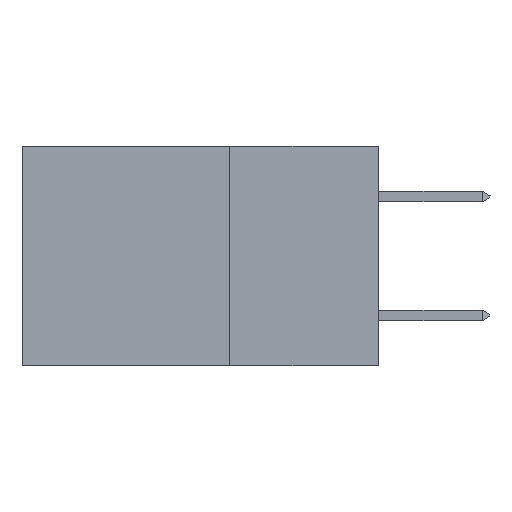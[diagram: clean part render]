
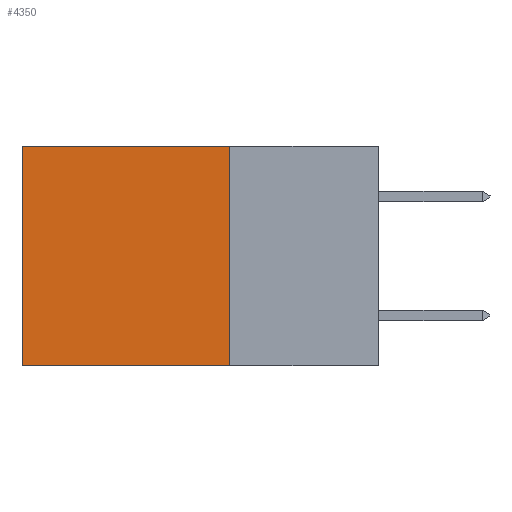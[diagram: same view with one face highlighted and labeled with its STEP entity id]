
A CAD part, left-side view. The second image highlights one B-rep face of the part: STEP entity #4350.
In plain terms, the highlighted planar face has unit normal (-1, 0, 0).
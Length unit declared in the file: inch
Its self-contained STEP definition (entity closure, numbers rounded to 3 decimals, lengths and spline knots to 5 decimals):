
#243 = EDGE_CURVE ( 'NONE', #7638, #7333, #8550, .T. ) ;
#1134 = LINE ( 'NONE', #7123, #10277 ) ;
#1399 = VERTEX_POINT ( 'NONE', #10328 ) ;
#1833 = EDGE_LOOP ( 'NONE', ( #2424, #3683, #6592, #6654 ) ) ;
#2219 = CARTESIAN_POINT ( 'NONE',  ( 0.2615, 0.25, -0.37 ) ) ;
#2424 = ORIENTED_EDGE ( 'NONE', *, *, #12618, .T. ) ;
#2612 = DIRECTION ( 'NONE',  ( 0., 1., 0. ) ) ;
#3199 = AXIS2_PLACEMENT_3D ( 'NONE', #2219, #3296, #6269 ) ;
#3251 = EDGE_CURVE ( 'NONE', #11670, #1399, #8200, .T. ) ;
#3296 = DIRECTION ( 'NONE',  ( 1., 0., 0. ) ) ;
#3599 = CARTESIAN_POINT ( 'NONE',  ( 0.2615, 0.25, -0.37 ) ) ;
#3664 = LINE ( 'NONE', #12708, #12023 ) ;
#3683 = ORIENTED_EDGE ( 'NONE', *, *, #243, .F. ) ;
#4350 = ADVANCED_FACE ( 'NONE', ( #5340 ), #7191, .F. ) ;
#5340 = FACE_OUTER_BOUND ( 'NONE', #1833, .T. ) ;
#6269 = DIRECTION ( 'NONE',  ( 0., 0., -1. ) ) ;
#6452 = EDGE_CURVE ( 'NONE', #11670, #7638, #3664, .T. ) ;
#6592 = ORIENTED_EDGE ( 'NONE', *, *, #6452, .F. ) ;
#6654 = ORIENTED_EDGE ( 'NONE', *, *, #3251, .T. ) ;
#7123 = CARTESIAN_POINT ( 'NONE',  ( 0.2615, 0.6, -0.37 ) ) ;
#7191 = PLANE ( 'NONE',  #3199 ) ;
#7274 = DIRECTION ( 'NONE',  ( 0., 1., 0. ) ) ;
#7333 = VERTEX_POINT ( 'NONE', #12725 ) ;
#7638 = VERTEX_POINT ( 'NONE', #12649 ) ;
#8139 = CARTESIAN_POINT ( 'NONE',  ( 0.2615, 0.25, 0. ) ) ;
#8200 = LINE ( 'NONE', #8139, #9602 ) ;
#8271 = CARTESIAN_POINT ( 'NONE',  ( 0.2615, 0.25, 0. ) ) ;
#8546 = DIRECTION ( 'NONE',  ( 0., 0., -1. ) ) ;
#8550 = LINE ( 'NONE', #3599, #11061 ) ;
#9349 = DIRECTION ( 'NONE',  ( 0., 0., -1. ) ) ;
#9602 = VECTOR ( 'NONE', #7274, 39.37008 ) ;
#10277 = VECTOR ( 'NONE', #9349, 39.37008 ) ;
#10328 = CARTESIAN_POINT ( 'NONE',  ( 0.2615, 0.6, 0. ) ) ;
#11061 = VECTOR ( 'NONE', #2612, 39.37008 ) ;
#11670 = VERTEX_POINT ( 'NONE', #8271 ) ;
#12023 = VECTOR ( 'NONE', #8546, 39.37008 ) ;
#12618 = EDGE_CURVE ( 'NONE', #1399, #7333, #1134, .T. ) ;
#12649 = CARTESIAN_POINT ( 'NONE',  ( 0.2615, 0.25, -0.37 ) ) ;
#12708 = CARTESIAN_POINT ( 'NONE',  ( 0.2615, 0.25, -0.37 ) ) ;
#12725 = CARTESIAN_POINT ( 'NONE',  ( 0.2615, 0.6, -0.37 ) ) ;
